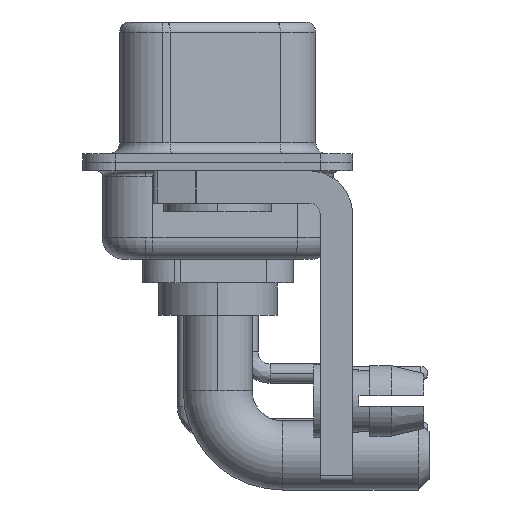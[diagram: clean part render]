
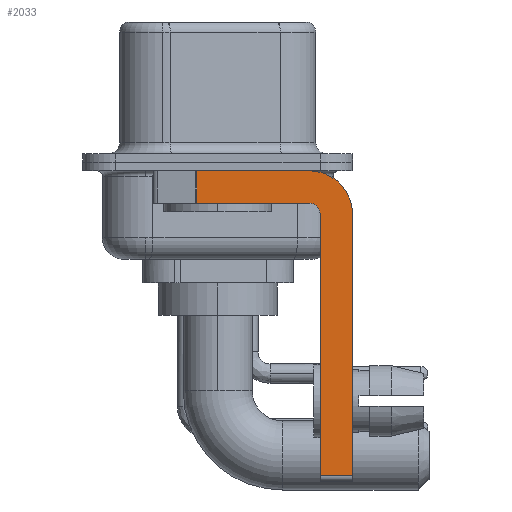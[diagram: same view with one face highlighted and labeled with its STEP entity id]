
A CAD part, left-side view. The second image highlights one B-rep face of the part: STEP entity #2033.
In plain terms, the highlighted planar face has unit normal (-1, 0, 0).
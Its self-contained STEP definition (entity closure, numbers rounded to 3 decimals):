
#140 = VECTOR ( 'NONE', #10390, 1000. ) ;
#821 = CARTESIAN_POINT ( 'NONE',  ( -2.9, -4.75, -2.4 ) ) ;
#968 = EDGE_CURVE ( 'NONE', #4772, #20253, #21995, .T. ) ;
#1192 = LINE ( 'NONE', #18495, #22232 ) ;
#1350 = EDGE_CURVE ( 'NONE', #10774, #3447, #6963, .T. ) ;
#2033 = ADVANCED_FACE ( 'NONE', ( #16581 ), #25627, .F. ) ;
#3447 = VERTEX_POINT ( 'NONE', #21801 ) ;
#3746 = CARTESIAN_POINT ( 'NONE',  ( -2.9, -4.75, -14.8 ) ) ;
#3797 = ORIENTED_EDGE ( 'NONE', *, *, #1350, .T. ) ;
#3956 = DIRECTION ( 'NONE',  ( 0., 0., -1. ) ) ;
#4319 = ORIENTED_EDGE ( 'NONE', *, *, #968, .F. ) ;
#4403 = VECTOR ( 'NONE', #26993, 1000. ) ;
#4772 = VERTEX_POINT ( 'NONE', #821 ) ;
#5644 = CARTESIAN_POINT ( 'NONE',  ( -2.9, -4.25, -2.4 ) ) ;
#5715 = EDGE_CURVE ( 'NONE', #12174, #3447, #12057, .T. ) ;
#6094 = DIRECTION ( 'NONE',  ( 1., 0., 0. ) ) ;
#6683 = CIRCLE ( 'NONE', #20296, 2. ) ;
#6843 = DIRECTION ( 'NONE',  ( 0., 0., -1. ) ) ;
#6863 = DIRECTION ( 'NONE',  ( -1., 0., 0. ) ) ;
#6963 = LINE ( 'NONE', #22138, #16151 ) ;
#8219 = ORIENTED_EDGE ( 'NONE', *, *, #5715, .F. ) ;
#8869 = LINE ( 'NONE', #24172, #12526 ) ;
#8996 = VECTOR ( 'NONE', #6843, 1000. ) ;
#9384 = EDGE_CURVE ( 'NONE', #10774, #4772, #22599, .T. ) ;
#9521 = ORIENTED_EDGE ( 'NONE', *, *, #9384, .F. ) ;
#9799 = AXIS2_PLACEMENT_3D ( 'NONE', #24021, #6863, #15539 ) ;
#10390 = DIRECTION ( 'NONE',  ( 0., 0., -1. ) ) ;
#10552 = CARTESIAN_POINT ( 'NONE',  ( -2.9, 0.978, -0.4 ) ) ;
#10661 = CARTESIAN_POINT ( 'NONE',  ( -2.9, -4.25, -2.4 ) ) ;
#10774 = VERTEX_POINT ( 'NONE', #17109 ) ;
#11001 = VERTEX_POINT ( 'NONE', #25254 ) ;
#11407 = CARTESIAN_POINT ( 'NONE',  ( -2.9, -6.25, -2.4 ) ) ;
#11825 = EDGE_CURVE ( 'NONE', #11001, #12174, #6683, .T. ) ;
#11828 = ORIENTED_EDGE ( 'NONE', *, *, #11825, .F. ) ;
#12022 = EDGE_LOOP ( 'NONE', ( #18551, #18079, #12355, #4319, #9521, #3797, #8219, #11828 ) ) ;
#12057 = LINE ( 'NONE', #11407, #8996 ) ;
#12174 = VERTEX_POINT ( 'NONE', #18814 ) ;
#12355 = ORIENTED_EDGE ( 'NONE', *, *, #25335, .F. ) ;
#12526 = VECTOR ( 'NONE', #15554, 1000. ) ;
#12990 = CARTESIAN_POINT ( 'NONE',  ( -2.9, 0.978, -1.9 ) ) ;
#15539 = DIRECTION ( 'NONE',  ( 0., 0., 1. ) ) ;
#15554 = DIRECTION ( 'NONE',  ( 0., 1., 0. ) ) ;
#16151 = VECTOR ( 'NONE', #19473, 1000. ) ;
#16242 = EDGE_CURVE ( 'NONE', #22757, #11001, #1192, .T. ) ;
#16581 = FACE_OUTER_BOUND ( 'NONE', #12022, .T. ) ;
#16769 = CARTESIAN_POINT ( 'NONE',  ( -2.9, 0.978, -1.9 ) ) ;
#17109 = CARTESIAN_POINT ( 'NONE',  ( -2.9, -4.75, -14.55 ) ) ;
#18079 = ORIENTED_EDGE ( 'NONE', *, *, #18088, .T. ) ;
#18088 = EDGE_CURVE ( 'NONE', #22757, #25295, #23269, .T. ) ;
#18495 = CARTESIAN_POINT ( 'NONE',  ( -2.9, 3., -0.4 ) ) ;
#18551 = ORIENTED_EDGE ( 'NONE', *, *, #16242, .F. ) ;
#18605 = CARTESIAN_POINT ( 'NONE',  ( -2.9, -4.25, -1.9 ) ) ;
#18814 = CARTESIAN_POINT ( 'NONE',  ( -2.9, -6.25, -2.4 ) ) ;
#19473 = DIRECTION ( 'NONE',  ( 0., -1., 0. ) ) ;
#20253 = VERTEX_POINT ( 'NONE', #18605 ) ;
#20296 = AXIS2_PLACEMENT_3D ( 'NONE', #10661, #6094, #21133 ) ;
#21027 = DIRECTION ( 'NONE',  ( 0., -1., 0. ) ) ;
#21133 = DIRECTION ( 'NONE',  ( 0., 0., -1. ) ) ;
#21374 = DIRECTION ( 'NONE',  ( 1., 0., 0. ) ) ;
#21801 = CARTESIAN_POINT ( 'NONE',  ( -2.9, -6.25, -14.55 ) ) ;
#21995 = CIRCLE ( 'NONE', #9799, 0.5 ) ;
#22138 = CARTESIAN_POINT ( 'NONE',  ( -2.9, -4.25, -14.55 ) ) ;
#22232 = VECTOR ( 'NONE', #21027, 1000. ) ;
#22599 = LINE ( 'NONE', #3746, #4403 ) ;
#22757 = VERTEX_POINT ( 'NONE', #10552 ) ;
#23269 = LINE ( 'NONE', #16769, #140 ) ;
#24021 = CARTESIAN_POINT ( 'NONE',  ( -2.9, -4.25, -2.4 ) ) ;
#24172 = CARTESIAN_POINT ( 'NONE',  ( -2.9, -4.25, -1.9 ) ) ;
#25254 = CARTESIAN_POINT ( 'NONE',  ( -2.9, -4.25, -0.4 ) ) ;
#25295 = VERTEX_POINT ( 'NONE', #12990 ) ;
#25335 = EDGE_CURVE ( 'NONE', #20253, #25295, #8869, .T. ) ;
#25627 = PLANE ( 'NONE',  #27160 ) ;
#26993 = DIRECTION ( 'NONE',  ( 0., 0., 1. ) ) ;
#27160 = AXIS2_PLACEMENT_3D ( 'NONE', #5644, #21374, #3956 ) ;
